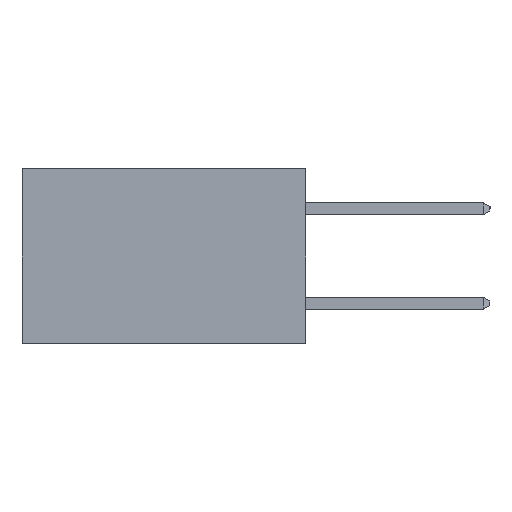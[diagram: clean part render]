
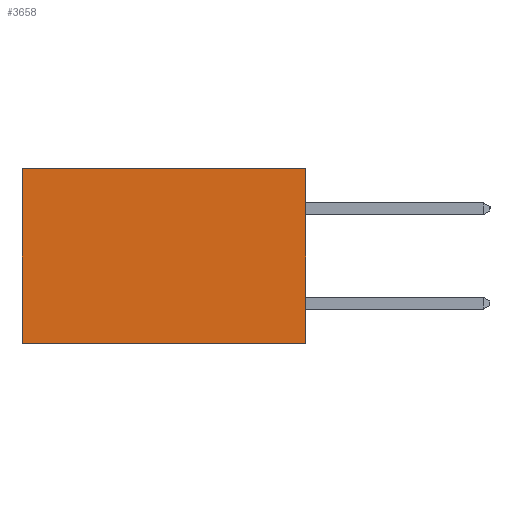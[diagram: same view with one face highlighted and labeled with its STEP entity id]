
A CAD part, left-side view. The second image highlights one B-rep face of the part: STEP entity #3658.
In plain terms, the highlighted planar face has unit normal (-1, 0, 0).
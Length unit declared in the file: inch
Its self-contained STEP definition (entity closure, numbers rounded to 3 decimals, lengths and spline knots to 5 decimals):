
#168 = CARTESIAN_POINT ( 'NONE',  ( 0.2615, 0.6, -0.37 ) ) ;
#198 = EDGE_CURVE ( 'NONE', #3632, #15768, #16237, .T. ) ;
#728 = CARTESIAN_POINT ( 'NONE',  ( 0.2615, 0., -0.37 ) ) ;
#966 = CARTESIAN_POINT ( 'NONE',  ( 0.2615, 0., -0.37 ) ) ;
#1326 = VECTOR ( 'NONE', #9454, 39.37008 ) ;
#1495 = CARTESIAN_POINT ( 'NONE',  ( 0.2615, 0., -0.37 ) ) ;
#1505 = EDGE_CURVE ( 'NONE', #7586, #3185, #8657, .T. ) ;
#2247 = EDGE_CURVE ( 'NONE', #3185, #15768, #8190, .T. ) ;
#2880 = FACE_OUTER_BOUND ( 'NONE', #13197, .T. ) ;
#3185 = VERTEX_POINT ( 'NONE', #1495 ) ;
#3510 = ORIENTED_EDGE ( 'NONE', *, *, #15626, .T. ) ;
#3632 = VERTEX_POINT ( 'NONE', #17555 ) ;
#3658 = ADVANCED_FACE ( 'NONE', ( #2880 ), #8799, .F. ) ;
#3665 = VECTOR ( 'NONE', #7455, 39.37008 ) ;
#5425 = ORIENTED_EDGE ( 'NONE', *, *, #1505, .F. ) ;
#6849 = DIRECTION ( 'NONE',  ( 1., 0., 0. ) ) ;
#6886 = CARTESIAN_POINT ( 'NONE',  ( 0.2615, 0., -0.37 ) ) ;
#6944 = DIRECTION ( 'NONE',  ( 0., 0., -1. ) ) ;
#7452 = VECTOR ( 'NONE', #12883, 39.37008 ) ;
#7455 = DIRECTION ( 'NONE',  ( 0., 0., -1. ) ) ;
#7586 = VERTEX_POINT ( 'NONE', #11493 ) ;
#7929 = ORIENTED_EDGE ( 'NONE', *, *, #198, .T. ) ;
#8190 = LINE ( 'NONE', #728, #10541 ) ;
#8657 = LINE ( 'NONE', #6886, #7452 ) ;
#8799 = PLANE ( 'NONE',  #10389 ) ;
#9454 = DIRECTION ( 'NONE',  ( 0., 1., 0. ) ) ;
#9631 = DIRECTION ( 'NONE',  ( 0., 1., 0. ) ) ;
#10389 = AXIS2_PLACEMENT_3D ( 'NONE', #966, #6849, #6944 ) ;
#10541 = VECTOR ( 'NONE', #9631, 39.37008 ) ;
#10917 = LINE ( 'NONE', #12171, #1326 ) ;
#11493 = CARTESIAN_POINT ( 'NONE',  ( 0.2615, 0., 0. ) ) ;
#12171 = CARTESIAN_POINT ( 'NONE',  ( 0.2615, 0., 0. ) ) ;
#12883 = DIRECTION ( 'NONE',  ( 0., 0., -1. ) ) ;
#13197 = EDGE_LOOP ( 'NONE', ( #7929, #16486, #5425, #3510 ) ) ;
#15626 = EDGE_CURVE ( 'NONE', #7586, #3632, #10917, .T. ) ;
#15768 = VERTEX_POINT ( 'NONE', #18898 ) ;
#16237 = LINE ( 'NONE', #168, #3665 ) ;
#16486 = ORIENTED_EDGE ( 'NONE', *, *, #2247, .F. ) ;
#17555 = CARTESIAN_POINT ( 'NONE',  ( 0.2615, 0.6, 0. ) ) ;
#18898 = CARTESIAN_POINT ( 'NONE',  ( 0.2615, 0.6, -0.37 ) ) ;
